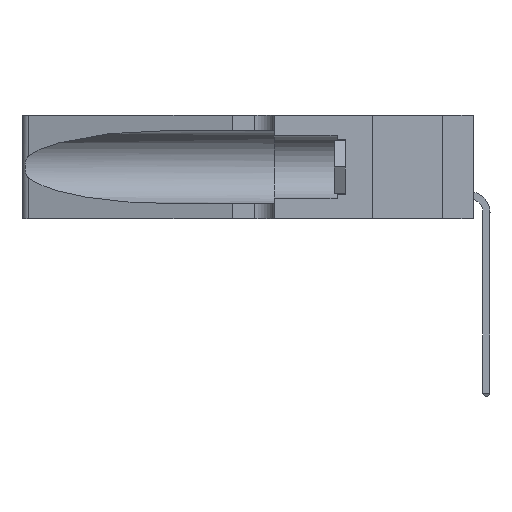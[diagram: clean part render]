
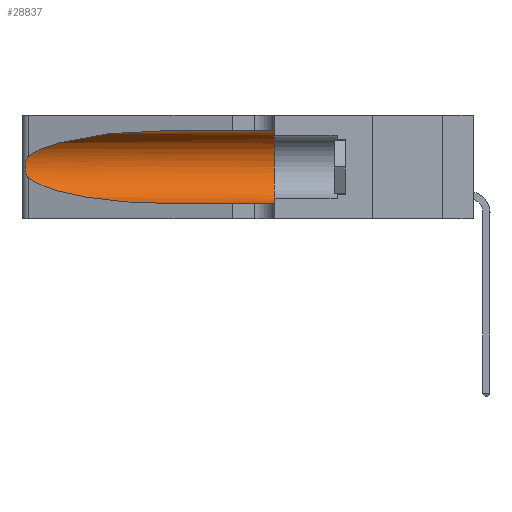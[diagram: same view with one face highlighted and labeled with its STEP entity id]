
A CAD part, left-side view. The second image highlights one B-rep face of the part: STEP entity #28837.
In plain terms, the highlighted cylindrical face has radius 3.308 mm (diameter 6.617 mm), a partial arc.
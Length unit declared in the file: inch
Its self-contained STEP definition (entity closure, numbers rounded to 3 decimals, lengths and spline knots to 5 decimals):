
#408 = DIRECTION ( 'NONE',  ( 0., 0., -1. ) ) ;
#929 = CARTESIAN_POINT ( 'NONE',  ( 0.26017, 1.23833, 0.17102 ) ) ;
#963 = CARTESIAN_POINT ( 'NONE',  ( 0.1305, 1.61858, 0.31525 ) ) ;
#1087 = DIRECTION ( 'NONE',  ( 0., -1., 0. ) ) ;
#1155 = EDGE_CURVE ( 'NONE', #17753, #4392, #8230, .T. ) ;
#1742 = LINE ( 'NONE', #11759, #16829 ) ;
#3951 = CARTESIAN_POINT ( 'NONE',  ( 0.25555, 1.22993, 0.14849 ) ) ;
#4014 = VERTEX_POINT ( 'NONE', #12718 ) ;
#4392 = VERTEX_POINT ( 'NONE', #24631 ) ;
#4491 = CARTESIAN_POINT ( 'NONE',  ( 0.2373, 1.15595, 0.08982 ) ) ;
#6414 = CARTESIAN_POINT ( 'NONE',  ( 0.25639, 1.23186, 0.15144 ) ) ;
#6517 = CARTESIAN_POINT ( 'NONE',  ( 0.25856, 1.23593, 0.16098 ) ) ;
#6869 = ORIENTED_EDGE ( 'NONE', *, *, #1155, .F. ) ;
#7099 = CARTESIAN_POINT ( 'NONE',  ( 0.25487, 1.22718, 0.22369 ) ) ;
#7647 = ORIENTED_EDGE ( 'NONE', *, *, #15100, .T. ) ;
#7682 = ORIENTED_EDGE ( 'NONE', *, *, #23508, .T. ) ;
#8230 = CIRCLE ( 'NONE', #11157, 0.13025 ) ;
#8266 = ORIENTED_EDGE ( 'NONE', *, *, #8656, .F. ) ;
#8656 = EDGE_CURVE ( 'NONE', #15339, #17753, #20819, .T. ) ;
#8965 = CARTESIAN_POINT ( 'NONE',  ( 0.25639, 1.23184, 0.21858 ) ) ;
#9684 = EDGE_CURVE ( 'NONE', #12336, #4392, #1742, .T. ) ;
#9858 = DIRECTION ( 'NONE',  ( 0., 1., 0. ) ) ;
#10069 = CARTESIAN_POINT ( 'NONE',  ( 0.1305, 0.35, 0.185 ) ) ;
#10146 = CARTESIAN_POINT ( 'NONE',  ( 0.18966, 0.96281, 0.05475 ) ) ;
#11157 = AXIS2_PLACEMENT_3D ( 'NONE', #10069, #9858, #25233 ) ;
#11310 = CARTESIAN_POINT ( 'NONE',  ( 0.1305, 0.72297, 0.31525 ) ) ;
#11759 = CARTESIAN_POINT ( 'NONE',  ( 0.1305, 1.61858, 0.05475 ) ) ;
#12246 = ORIENTED_EDGE ( 'NONE', *, *, #18638, .T. ) ;
#12336 = VERTEX_POINT ( 'NONE', #21926 ) ;
#12718 = CARTESIAN_POINT ( 'NONE',  ( 0.25487, 1.22718, 0.22369 ) ) ;
#13386 = AXIS2_PLACEMENT_3D ( 'NONE', #15906, #23164, #408 ) ;
#13990 = CARTESIAN_POINT ( 'NONE',  ( 0.18966, 0.96281, 0.31525 ) ) ;
#14084 = CARTESIAN_POINT ( 'NONE',  ( 0.26075, 1.23896, 0.19203 ) ) ;
#14162 = VECTOR ( 'NONE', #1087, 39.37008 ) ;
#15100 = EDGE_CURVE ( 'NONE', #4014, #25450, #19374, .T. ) ;
#15339 = VERTEX_POINT ( 'NONE', #19787 ) ;
#15906 = CARTESIAN_POINT ( 'NONE',  ( 0.1305, 1.61858, 0.185 ) ) ;
#16829 = VECTOR ( 'NONE', #31925, 39.37008 ) ;
#17674 = CARTESIAN_POINT ( 'NONE',  ( 0.1305, 0.72297, 0.05475 ) ) ;
#17753 = VERTEX_POINT ( 'NONE', #29478 ) ;
#18638 = EDGE_CURVE ( 'NONE', #25450, #12336, #21170, .T. ) ;
#19151 = CARTESIAN_POINT ( 'NONE',  ( 0.25854, 1.2359, 0.20912 ) ) ;
#19173 = CARTESIAN_POINT ( 'NONE',  ( 0.25487, 1.22718, 0.14631 ) ) ;
#19374 = B_SPLINE_CURVE_WITH_KNOTS ( 'NONE', 3,
 ( #7099, #30453, #8965, #29158, #19151, #31450, #14084, #21551, #929, #6517, #26409, #6414, #3951, #31680 ),
 .UNSPECIFIED., .F., .F.,
 ( 4, 2, 2, 2, 2, 2, 4 ),
 ( 0., 0.00027, 0.00053, 0.00107, 0.0016, 0.00187, 0.00214 ),
 .UNSPECIFIED. ) ;
#19787 = CARTESIAN_POINT ( 'NONE',  ( 0.1305, 0.72297, 0.31525 ) ) ;
#20819 = LINE ( 'NONE', #963, #14162 ) ;
#21170 =( BOUNDED_CURVE ( )  B_SPLINE_CURVE ( 3, ( #24658, #4491, #10146, #17674 ),
 .UNSPECIFIED., .F., .F. ) 
 B_SPLINE_CURVE_WITH_KNOTS ( ( 4, 4 ),
 ( 3.44316, 4.71239 ),
 .UNSPECIFIED. ) 
 CURVE ( )  GEOMETRIC_REPRESENTATION_ITEM ( )  RATIONAL_B_SPLINE_CURVE ( ( 1., 0.87, 0.87, 1. ) ) 
 REPRESENTATION_ITEM ( '' )  );
#21551 = CARTESIAN_POINT ( 'NONE',  ( 0.26075, 1.23896, 0.178 ) ) ;
#21926 = CARTESIAN_POINT ( 'NONE',  ( 0.1305, 0.72297, 0.05475 ) ) ;
#23164 = DIRECTION ( 'NONE',  ( 0., -1., 0. ) ) ;
#23181 = FACE_OUTER_BOUND ( 'NONE', #30981, .T. ) ;
#23508 = EDGE_CURVE ( 'NONE', #15339, #4014, #30424, .T. ) ;
#24631 = CARTESIAN_POINT ( 'NONE',  ( 0.1305, 0.35, 0.05475 ) ) ;
#24658 = CARTESIAN_POINT ( 'NONE',  ( 0.25487, 1.22718, 0.14631 ) ) ;
#24769 = CARTESIAN_POINT ( 'NONE',  ( 0.2373, 1.15595, 0.28018 ) ) ;
#25177 = CYLINDRICAL_SURFACE ( 'NONE', #13386, 0.13025 ) ;
#25233 = DIRECTION ( 'NONE',  ( 0., 0., 1. ) ) ;
#25450 = VERTEX_POINT ( 'NONE', #19173 ) ;
#26409 = CARTESIAN_POINT ( 'NONE',  ( 0.25789, 1.23486, 0.15765 ) ) ;
#28103 = CARTESIAN_POINT ( 'NONE',  ( 0.25487, 1.22718, 0.22369 ) ) ;
#28818 = ORIENTED_EDGE ( 'NONE', *, *, #9684, .T. ) ;
#28837 = ADVANCED_FACE ( 'NONE', ( #23181 ), #25177, .F. ) ;
#29158 = CARTESIAN_POINT ( 'NONE',  ( 0.25787, 1.23484, 0.2124 ) ) ;
#29478 = CARTESIAN_POINT ( 'NONE',  ( 0.1305, 0.35, 0.31525 ) ) ;
#30424 =( BOUNDED_CURVE ( )  B_SPLINE_CURVE ( 3, ( #11310, #13990, #24769, #28103 ),
 .UNSPECIFIED., .F., .F. ) 
 B_SPLINE_CURVE_WITH_KNOTS ( ( 4, 4 ),
 ( 1.5708, 2.84003 ),
 .UNSPECIFIED. ) 
 CURVE ( )  GEOMETRIC_REPRESENTATION_ITEM ( )  RATIONAL_B_SPLINE_CURVE ( ( 1., 0.87, 0.87, 1. ) ) 
 REPRESENTATION_ITEM ( '' )  );
#30453 = CARTESIAN_POINT ( 'NONE',  ( 0.25555, 1.22994, 0.2215 ) ) ;
#30981 = EDGE_LOOP ( 'NONE', ( #7682, #7647, #12246, #28818, #6869, #8266 ) ) ;
#31450 = CARTESIAN_POINT ( 'NONE',  ( 0.26018, 1.23835, 0.19895 ) ) ;
#31680 = CARTESIAN_POINT ( 'NONE',  ( 0.25487, 1.22718, 0.14631 ) ) ;
#31925 = DIRECTION ( 'NONE',  ( 0., -1., 0. ) ) ;
